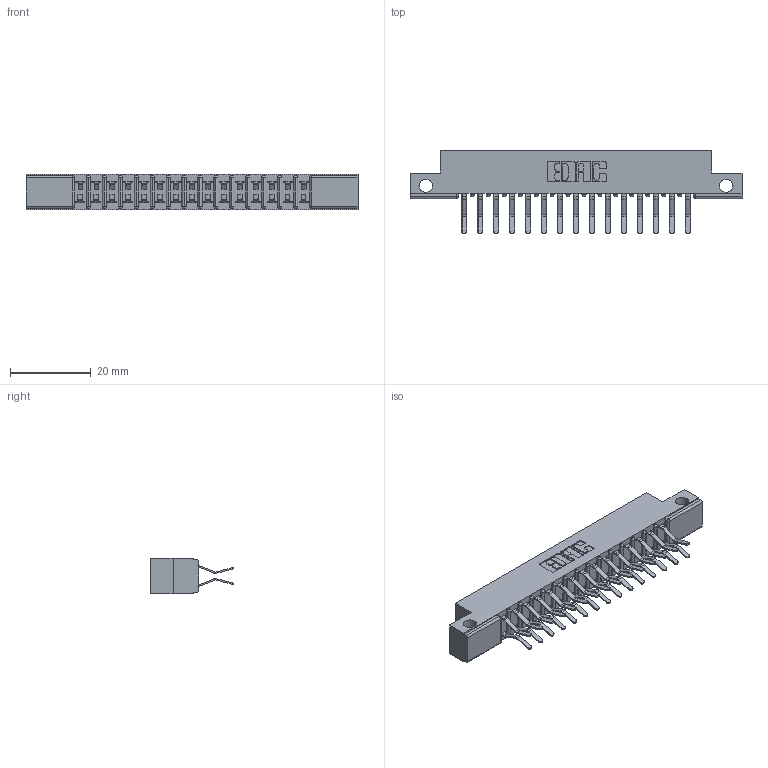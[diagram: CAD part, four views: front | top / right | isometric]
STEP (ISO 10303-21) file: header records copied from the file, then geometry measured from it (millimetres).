
FILE_DESCRIPTION (( 'STEP AP203' ), '1' );
FILE_NAME ('357-030-560-212.STEP', '2019-09-18T01:02:07', ( '' ), ( '' ), 'SwSTEP 2.0', 'SolidWorks 2016', '' );
FILE_SCHEMA (( 'CONFIG_CONTROL_DESIGN' ));
Length unit declared in the file: inch
Products named in the file (3): 357-030-560-212; 307-290-001_560; 307 Part_.128 Dia Side Mounting Holes
Assembly tree (31 placements, depth 2):
  357-030-560-212
    307 Part_.128 Dia Side Mounting Holes
    307-290-001_560  x30
Bounding box: 82.45 x 20.73 x 8.71 mm (x, y, z)
Volume: 5355.3 mm3; surface area: 9182.5 mm2
Topology: 31 solids, 31 shells, 1634 faces, 4583 edges, 2970 vertices
Faces by surface type: plane 1060, cylinder 542, sphere 32
Entity records: 16774 total; most frequent: CARTESIAN_POINT 2751, ORIENTED_EDGE 2722, DIRECTION 2707, EDGE_CURVE 1361, LINE 1031, VECTOR 1031, VERTEX_POINT 882, AXIS2_PLACEMENT_3D 838
